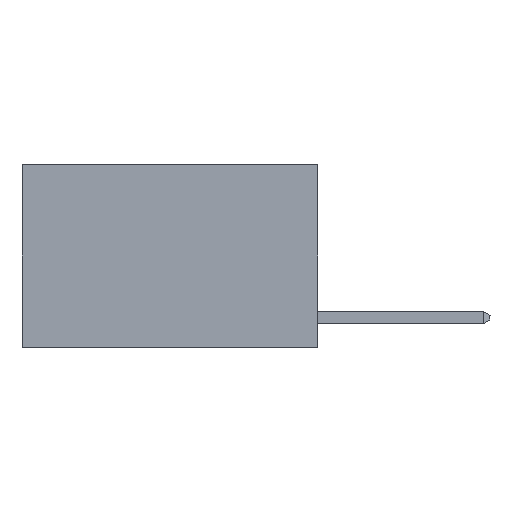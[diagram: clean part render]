
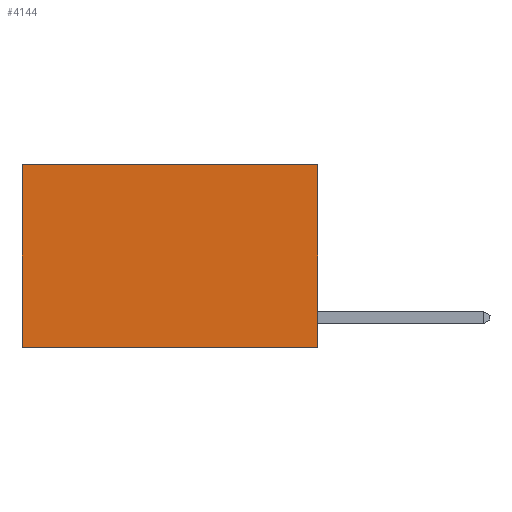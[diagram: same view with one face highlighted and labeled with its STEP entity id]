
A CAD part, left-side view. The second image highlights one B-rep face of the part: STEP entity #4144.
In plain terms, the highlighted planar face has unit normal (-1, 0, 0).
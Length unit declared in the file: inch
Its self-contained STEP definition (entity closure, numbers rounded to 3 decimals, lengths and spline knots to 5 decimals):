
#58 = EDGE_CURVE ( 'NONE', #15949, #20042, #18289, .T. ) ;
#459 = ORIENTED_EDGE ( 'NONE', *, *, #58, .F. ) ;
#622 = LINE ( 'NONE', #9871, #7977 ) ;
#1344 = AXIS2_PLACEMENT_3D ( 'NONE', #14007, #1618, #14087 ) ;
#1405 = VECTOR ( 'NONE', #21100, 39.37008 ) ;
#1430 = CARTESIAN_POINT ( 'NONE',  ( 0.2625, 0.6, 0. ) ) ;
#1567 = ORIENTED_EDGE ( 'NONE', *, *, #11615, .T. ) ;
#1618 = DIRECTION ( 'NONE',  ( 1., 0., 0. ) ) ;
#2271 = EDGE_CURVE ( 'NONE', #15949, #15664, #11309, .T. ) ;
#2296 = ORIENTED_EDGE ( 'NONE', *, *, #6140, .F. ) ;
#4144 = ADVANCED_FACE ( 'NONE', ( #7070 ), #12318, .F. ) ;
#4786 = VECTOR ( 'NONE', #22524, 39.37008 ) ;
#5221 = CARTESIAN_POINT ( 'NONE',  ( 0.2625, 0., 0. ) ) ;
#5695 = CARTESIAN_POINT ( 'NONE',  ( 0.2625, 0., -0.37 ) ) ;
#5714 = CARTESIAN_POINT ( 'NONE',  ( 0.2625, 0., 0. ) ) ;
#6140 = EDGE_CURVE ( 'NONE', #20042, #16427, #622, .T. ) ;
#7024 = DIRECTION ( 'NONE',  ( 0., 1., 0. ) ) ;
#7070 = FACE_OUTER_BOUND ( 'NONE', #8933, .T. ) ;
#7149 = CARTESIAN_POINT ( 'NONE',  ( 0.2625, 0.6, 0. ) ) ;
#7722 = CARTESIAN_POINT ( 'NONE',  ( 0.2625, 0.6, -0.37 ) ) ;
#7977 = VECTOR ( 'NONE', #20328, 39.37008 ) ;
#8933 = EDGE_LOOP ( 'NONE', ( #1567, #2296, #459, #19488 ) ) ;
#9871 = CARTESIAN_POINT ( 'NONE',  ( 0.2625, 0., -0.37 ) ) ;
#11309 = LINE ( 'NONE', #5221, #15428 ) ;
#11615 = EDGE_CURVE ( 'NONE', #15664, #16427, #13952, .T. ) ;
#12318 = PLANE ( 'NONE',  #1344 ) ;
#13952 = LINE ( 'NONE', #7149, #1405 ) ;
#14007 = CARTESIAN_POINT ( 'NONE',  ( 0.2625, 0., 0. ) ) ;
#14087 = DIRECTION ( 'NONE',  ( 0., 0., -1. ) ) ;
#14720 = CARTESIAN_POINT ( 'NONE',  ( 0.2625, 0., 0. ) ) ;
#15428 = VECTOR ( 'NONE', #7024, 39.37008 ) ;
#15664 = VERTEX_POINT ( 'NONE', #1430 ) ;
#15949 = VERTEX_POINT ( 'NONE', #14720 ) ;
#16427 = VERTEX_POINT ( 'NONE', #7722 ) ;
#18289 = LINE ( 'NONE', #5714, #4786 ) ;
#19488 = ORIENTED_EDGE ( 'NONE', *, *, #2271, .T. ) ;
#20042 = VERTEX_POINT ( 'NONE', #5695 ) ;
#20328 = DIRECTION ( 'NONE',  ( 0., 1., 0. ) ) ;
#21100 = DIRECTION ( 'NONE',  ( 0., 0., -1. ) ) ;
#22524 = DIRECTION ( 'NONE',  ( 0., 0., -1. ) ) ;
